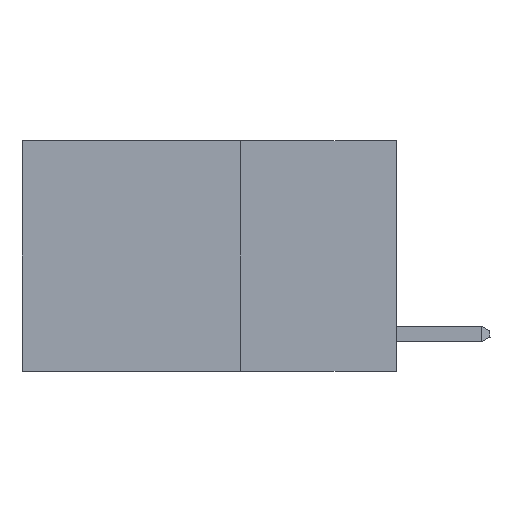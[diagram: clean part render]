
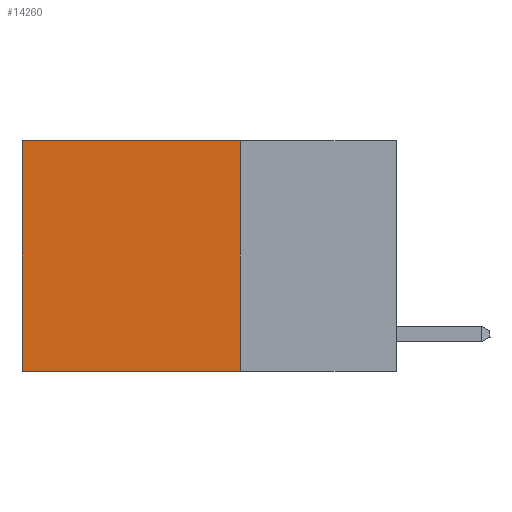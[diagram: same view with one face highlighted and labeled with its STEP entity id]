
A CAD part, left-side view. The second image highlights one B-rep face of the part: STEP entity #14260.
In plain terms, the highlighted planar face has unit normal (-1, 0, 0).
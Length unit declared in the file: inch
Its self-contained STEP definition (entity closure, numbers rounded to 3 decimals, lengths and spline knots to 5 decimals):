
#443 = EDGE_CURVE ( 'NONE', #6033, #3162, #17309, .T. ) ;
#463 = LINE ( 'NONE', #16151, #8456 ) ;
#1660 = DIRECTION ( 'NONE',  ( 0., 0., -1. ) ) ;
#2122 = AXIS2_PLACEMENT_3D ( 'NONE', #3489, #14135, #5136 ) ;
#3162 = VERTEX_POINT ( 'NONE', #4040 ) ;
#3489 = CARTESIAN_POINT ( 'NONE',  ( 0.2625, 0.25, 0. ) ) ;
#3510 = EDGE_CURVE ( 'NONE', #10975, #6033, #463, .T. ) ;
#4040 = CARTESIAN_POINT ( 'NONE',  ( 0.2625, 0.6, -0.37 ) ) ;
#4968 = DIRECTION ( 'NONE',  ( 0., 0., -1. ) ) ;
#5136 = DIRECTION ( 'NONE',  ( 0., 0., -1. ) ) ;
#6014 = EDGE_CURVE ( 'NONE', #19536, #3162, #6786, .T. ) ;
#6033 = VERTEX_POINT ( 'NONE', #13429 ) ;
#6786 = LINE ( 'NONE', #17802, #7728 ) ;
#7711 = ORIENTED_EDGE ( 'NONE', *, *, #3510, .T. ) ;
#7728 = VECTOR ( 'NONE', #16314, 39.37008 ) ;
#7853 = CARTESIAN_POINT ( 'NONE',  ( 0.2625, 0.25, 0. ) ) ;
#8002 = CARTESIAN_POINT ( 'NONE',  ( 0.2625, 0.25, 0. ) ) ;
#8066 = ORIENTED_EDGE ( 'NONE', *, *, #18581, .F. ) ;
#8456 = VECTOR ( 'NONE', #8799, 39.37008 ) ;
#8754 = FACE_OUTER_BOUND ( 'NONE', #14351, .T. ) ;
#8799 = DIRECTION ( 'NONE',  ( 0., 1., 0. ) ) ;
#9456 = VECTOR ( 'NONE', #4968, 39.37008 ) ;
#10199 = ORIENTED_EDGE ( 'NONE', *, *, #6014, .F. ) ;
#10975 = VERTEX_POINT ( 'NONE', #7853 ) ;
#11631 = LINE ( 'NONE', #8002, #18106 ) ;
#12501 = CARTESIAN_POINT ( 'NONE',  ( 0.2625, 0.25, -0.37 ) ) ;
#13429 = CARTESIAN_POINT ( 'NONE',  ( 0.2625, 0.6, 0. ) ) ;
#14135 = DIRECTION ( 'NONE',  ( 1., 0., 0. ) ) ;
#14260 = ADVANCED_FACE ( 'NONE', ( #8754 ), #18502, .F. ) ;
#14351 = EDGE_LOOP ( 'NONE', ( #14508, #10199, #8066, #7711 ) ) ;
#14508 = ORIENTED_EDGE ( 'NONE', *, *, #443, .T. ) ;
#16151 = CARTESIAN_POINT ( 'NONE',  ( 0.2625, 0.25, 0. ) ) ;
#16314 = DIRECTION ( 'NONE',  ( 0., 1., 0. ) ) ;
#17309 = LINE ( 'NONE', #18127, #9456 ) ;
#17802 = CARTESIAN_POINT ( 'NONE',  ( 0.2625, 0.25, -0.37 ) ) ;
#18106 = VECTOR ( 'NONE', #1660, 39.37008 ) ;
#18127 = CARTESIAN_POINT ( 'NONE',  ( 0.2625, 0.6, 0. ) ) ;
#18502 = PLANE ( 'NONE',  #2122 ) ;
#18581 = EDGE_CURVE ( 'NONE', #10975, #19536, #11631, .T. ) ;
#19536 = VERTEX_POINT ( 'NONE', #12501 ) ;
